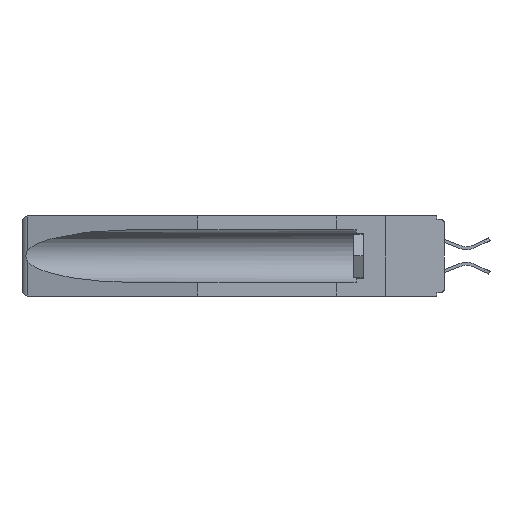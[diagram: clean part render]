
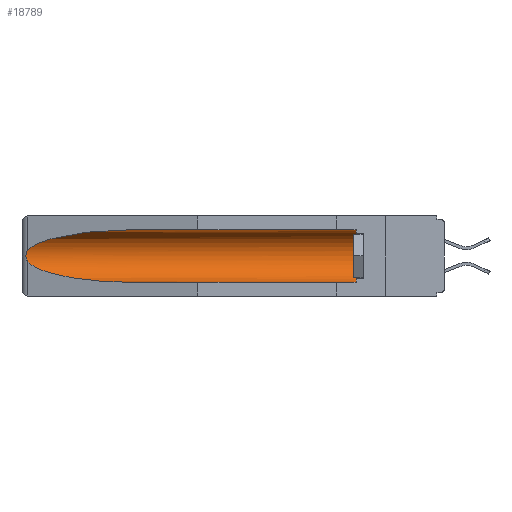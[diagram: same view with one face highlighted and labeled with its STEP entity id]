
A CAD part, left-side view. The second image highlights one B-rep face of the part: STEP entity #18789.
In plain terms, the highlighted cylindrical face has radius 2.857 mm (diameter 5.715 mm), a partial arc.
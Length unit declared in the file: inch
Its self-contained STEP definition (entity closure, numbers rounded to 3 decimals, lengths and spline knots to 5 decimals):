
#1027 = VERTEX_POINT ( 'NONE', #2607 ) ;
#1247 = VECTOR ( 'NONE', #17675, 39.37008 ) ;
#1556 = CARTESIAN_POINT ( 'NONE',  ( 0.25451, 1.48313, -0.24835 ) ) ;
#1912 = AXIS2_PLACEMENT_3D ( 'NONE', #3452, #20227, #12797 ) ;
#2607 = CARTESIAN_POINT ( 'NONE',  ( 0.155, 1.07973, -0.059 ) ) ;
#2837 = CARTESIAN_POINT ( 'NONE',  ( 0.26537, 1.52718, -0.14972 ) ) ;
#3171 = ORIENTED_EDGE ( 'NONE', *, *, #6428, .T. ) ;
#3452 = CARTESIAN_POINT ( 'NONE',  ( 0.155, 0.126, -0.1715 ) ) ;
#3549 = EDGE_LOOP ( 'NONE', ( #11426, #17699, #12586, #9991, #3171, #11897 ) ) ;
#4232 = EDGE_CURVE ( 'NONE', #22184, #23123, #5899, .T. ) ;
#4331 = FACE_OUTER_BOUND ( 'NONE', #3549, .T. ) ;
#4502 =( BOUNDED_CURVE ( )  B_SPLINE_CURVE ( 3, ( #8149, #22667, #8063, #7913 ),
 .UNSPECIFIED., .F., .F. ) 
 B_SPLINE_CURVE_WITH_KNOTS ( ( 4, 4 ),
 ( 4.71239, 6.08839 ),
 .UNSPECIFIED. ) 
 CURVE ( )  GEOMETRIC_REPRESENTATION_ITEM ( )  RATIONAL_B_SPLINE_CURVE ( ( 1., 0.848, 0.848, 1. ) ) 
 REPRESENTATION_ITEM ( '' )  );
#4704 = CARTESIAN_POINT ( 'NONE',  ( 0.2673, 1.53269, -0.17917 ) ) ;
#5730 = DIRECTION ( 'NONE',  ( 0., 1., 0. ) ) ;
#5899 = LINE ( 'NONE', #19090, #11114 ) ;
#6295 = CARTESIAN_POINT ( 'NONE',  ( 0.26537, 1.52718, -0.19328 ) ) ;
#6427 = CARTESIAN_POINT ( 'NONE',  ( 0.26537, 1.52718, -0.19328 ) ) ;
#6428 = EDGE_CURVE ( 'NONE', #22184, #17116, #23008, .T. ) ;
#6582 = CARTESIAN_POINT ( 'NONE',  ( 0.26655, 1.53094, -0.18657 ) ) ;
#7913 = CARTESIAN_POINT ( 'NONE',  ( 0.26537, 1.52718, -0.14972 ) ) ;
#8063 = CARTESIAN_POINT ( 'NONE',  ( 0.25451, 1.48313, -0.09465 ) ) ;
#8149 = CARTESIAN_POINT ( 'NONE',  ( 0.155, 1.07973, -0.059 ) ) ;
#8522 = CARTESIAN_POINT ( 'NONE',  ( 0.26597, 1.5296, -0.19026 ) ) ;
#9307 = CARTESIAN_POINT ( 'NONE',  ( 0.155, -0.30754, -0.1715 ) ) ;
#9991 = ORIENTED_EDGE ( 'NONE', *, *, #4232, .F. ) ;
#10438 = EDGE_CURVE ( 'NONE', #19192, #23006, #14991, .T. ) ;
#11114 = VECTOR ( 'NONE', #13357, 39.37008 ) ;
#11426 = ORIENTED_EDGE ( 'NONE', *, *, #14298, .T. ) ;
#11678 = EDGE_CURVE ( 'NONE', #23006, #23123, #14233, .T. ) ;
#11897 = ORIENTED_EDGE ( 'NONE', *, *, #13525, .T. ) ;
#11976 = CARTESIAN_POINT ( 'NONE',  ( 0.2673, 1.5327, -0.16383 ) ) ;
#12211 = CARTESIAN_POINT ( 'NONE',  ( 0.155, -0.30754, -0.059 ) ) ;
#12586 = ORIENTED_EDGE ( 'NONE', *, *, #11678, .T. ) ;
#12797 = DIRECTION ( 'NONE',  ( 0., 0., 1. ) ) ;
#13357 = DIRECTION ( 'NONE',  ( 0., 1., 0. ) ) ;
#13525 = EDGE_CURVE ( 'NONE', #17116, #1027, #14977, .T. ) ;
#13985 = CYLINDRICAL_SURFACE ( 'NONE', #21654, 0.1125 ) ;
#14090 = CARTESIAN_POINT ( 'NONE',  ( 0.26597, 1.52961, -0.15275 ) ) ;
#14233 =( BOUNDED_CURVE ( )  B_SPLINE_CURVE ( 3, ( #22012, #1556, #18440, #14603 ),
 .UNSPECIFIED., .F., .F. ) 
 B_SPLINE_CURVE_WITH_KNOTS ( ( 4, 4 ),
 ( 0.1948, 1.5708 ),
 .UNSPECIFIED. ) 
 CURVE ( )  GEOMETRIC_REPRESENTATION_ITEM ( )  RATIONAL_B_SPLINE_CURVE ( ( 1., 0.848, 0.848, 1. ) ) 
 REPRESENTATION_ITEM ( '' )  );
#14298 = EDGE_CURVE ( 'NONE', #1027, #19192, #4502, .T. ) ;
#14603 = CARTESIAN_POINT ( 'NONE',  ( 0.155, 1.07973, -0.284 ) ) ;
#14604 = CARTESIAN_POINT ( 'NONE',  ( 0.155, 0.126, -0.059 ) ) ;
#14720 = CARTESIAN_POINT ( 'NONE',  ( 0.155, 0.126, -0.284 ) ) ;
#14977 = LINE ( 'NONE', #12211, #1247 ) ;
#14991 = B_SPLINE_CURVE_WITH_KNOTS ( 'NONE', 3,
 ( #2837, #14090, #17618, #11976, #19392, #19466, #4704, #6582, #8522, #6427 ),
 .UNSPECIFIED., .F., .F.,
 ( 4, 2, 2, 2, 4 ),
 ( 0., 0.00029, 0.00058, 0.00087, 0.00117 ),
 .UNSPECIFIED. ) ;
#16819 = CARTESIAN_POINT ( 'NONE',  ( 0.155, 1.07973, -0.284 ) ) ;
#16869 = CARTESIAN_POINT ( 'NONE',  ( 0.26537, 1.52718, -0.14972 ) ) ;
#17116 = VERTEX_POINT ( 'NONE', #14604 ) ;
#17618 = CARTESIAN_POINT ( 'NONE',  ( 0.26654, 1.53092, -0.15636 ) ) ;
#17675 = DIRECTION ( 'NONE',  ( 0., 1., 0. ) ) ;
#17699 = ORIENTED_EDGE ( 'NONE', *, *, #10438, .T. ) ;
#18440 = CARTESIAN_POINT ( 'NONE',  ( 0.21114, 1.30732, -0.284 ) ) ;
#18789 = ADVANCED_FACE ( 'NONE', ( #4331 ), #13985, .F. ) ;
#19090 = CARTESIAN_POINT ( 'NONE',  ( 0.155, -0.30754, -0.284 ) ) ;
#19192 = VERTEX_POINT ( 'NONE', #16869 ) ;
#19392 = CARTESIAN_POINT ( 'NONE',  ( 0.2675, 1.53308, -0.16763 ) ) ;
#19466 = CARTESIAN_POINT ( 'NONE',  ( 0.2675, 1.53308, -0.17534 ) ) ;
#20227 = DIRECTION ( 'NONE',  ( 0., -1., 0. ) ) ;
#20807 = DIRECTION ( 'NONE',  ( 0., 0., 1. ) ) ;
#21654 = AXIS2_PLACEMENT_3D ( 'NONE', #9307, #5730, #20807 ) ;
#22012 = CARTESIAN_POINT ( 'NONE',  ( 0.26537, 1.52718, -0.19328 ) ) ;
#22184 = VERTEX_POINT ( 'NONE', #14720 ) ;
#22667 = CARTESIAN_POINT ( 'NONE',  ( 0.21114, 1.30732, -0.059 ) ) ;
#23006 = VERTEX_POINT ( 'NONE', #6295 ) ;
#23008 = CIRCLE ( 'NONE', #1912, 0.1125 ) ;
#23123 = VERTEX_POINT ( 'NONE', #16819 ) ;
